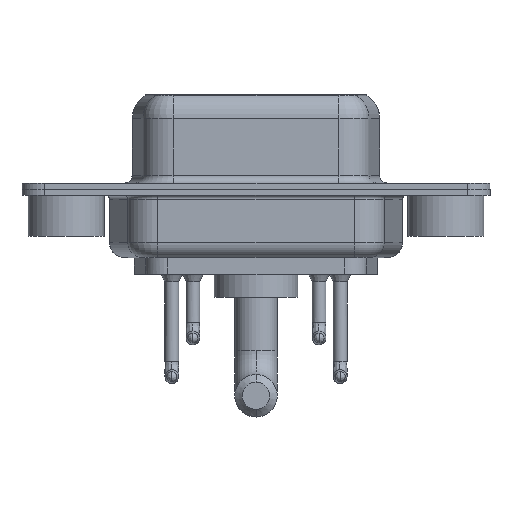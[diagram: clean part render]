
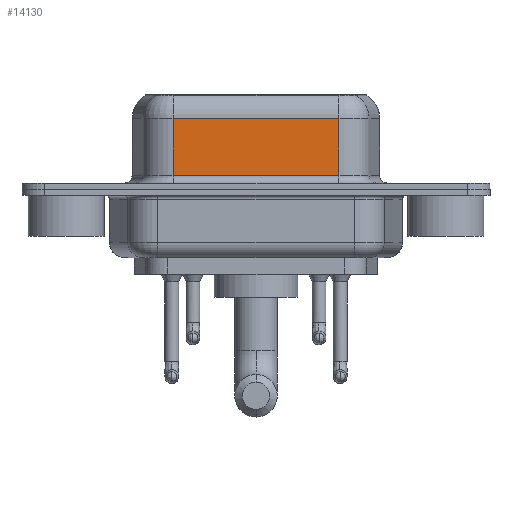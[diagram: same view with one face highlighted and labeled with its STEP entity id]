
A CAD part, front view. The second image highlights one B-rep face of the part: STEP entity #14130.
In plain terms, the highlighted planar face has unit normal (0, -1, 0).
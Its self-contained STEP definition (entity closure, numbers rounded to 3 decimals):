
#596 = CARTESIAN_POINT ( 'NONE',  ( 17.962, -3.95, 6.4 ) ) ;
#845 = LINE ( 'NONE', #596, #15877 ) ;
#1165 = VERTEX_POINT ( 'NONE', #11878 ) ;
#1369 = CARTESIAN_POINT ( 'NONE',  ( 7.038, -3.95, 4.65 ) ) ;
#1738 = CARTESIAN_POINT ( 'NONE',  ( 17.962, -3.95, 0.9 ) ) ;
#1974 = DIRECTION ( 'NONE',  ( 1., 0., 0. ) ) ;
#2102 = CARTESIAN_POINT ( 'NONE',  ( 7.038, -3.95, 6.4 ) ) ;
#2283 = AXIS2_PLACEMENT_3D ( 'NONE', #12179, #11020, #6033 ) ;
#3020 = LINE ( 'NONE', #2102, #13993 ) ;
#3368 = ORIENTED_EDGE ( 'NONE', *, *, #14687, .T. ) ;
#4506 = DIRECTION ( 'NONE',  ( -1., 0., 0. ) ) ;
#5339 = EDGE_CURVE ( 'NONE', #8862, #1165, #3020, .T. ) ;
#6033 = DIRECTION ( 'NONE',  ( -1., 0., 0. ) ) ;
#6567 = LINE ( 'NONE', #11621, #7033 ) ;
#6743 = EDGE_CURVE ( 'NONE', #1165, #12368, #15842, .T. ) ;
#7033 = VECTOR ( 'NONE', #4506, 1000. ) ;
#7112 = DIRECTION ( 'NONE',  ( 0., 0., -1. ) ) ;
#7223 = EDGE_CURVE ( 'NONE', #14451, #12368, #845, .T. ) ;
#8008 = CARTESIAN_POINT ( 'NONE',  ( 17.962, -3.95, 4.65 ) ) ;
#8862 = VERTEX_POINT ( 'NONE', #1369 ) ;
#9477 = ORIENTED_EDGE ( 'NONE', *, *, #5339, .T. ) ;
#10897 = ORIENTED_EDGE ( 'NONE', *, *, #7223, .F. ) ;
#11020 = DIRECTION ( 'NONE',  ( 0., 1., 0. ) ) ;
#11094 = FACE_OUTER_BOUND ( 'NONE', #14323, .T. ) ;
#11621 = CARTESIAN_POINT ( 'NONE',  ( 17.962, -3.95, 4.65 ) ) ;
#11878 = CARTESIAN_POINT ( 'NONE',  ( 7.038, -3.95, 0.9 ) ) ;
#12179 = CARTESIAN_POINT ( 'NONE',  ( 17.962, -3.95, 6.4 ) ) ;
#12368 = VERTEX_POINT ( 'NONE', #13352 ) ;
#13352 = CARTESIAN_POINT ( 'NONE',  ( 17.962, -3.95, 0.9 ) ) ;
#13356 = DIRECTION ( 'NONE',  ( 0., 0., -1. ) ) ;
#13838 = ORIENTED_EDGE ( 'NONE', *, *, #6743, .T. ) ;
#13993 = VECTOR ( 'NONE', #13356, 1000. ) ;
#14130 = ADVANCED_FACE ( 'NONE', ( #11094 ), #16122, .F. ) ;
#14323 = EDGE_LOOP ( 'NONE', ( #10897, #3368, #9477, #13838 ) ) ;
#14451 = VERTEX_POINT ( 'NONE', #8008 ) ;
#14687 = EDGE_CURVE ( 'NONE', #14451, #8862, #6567, .T. ) ;
#15608 = VECTOR ( 'NONE', #1974, 1000. ) ;
#15842 = LINE ( 'NONE', #1738, #15608 ) ;
#15877 = VECTOR ( 'NONE', #7112, 1000. ) ;
#16122 = PLANE ( 'NONE',  #2283 ) ;
